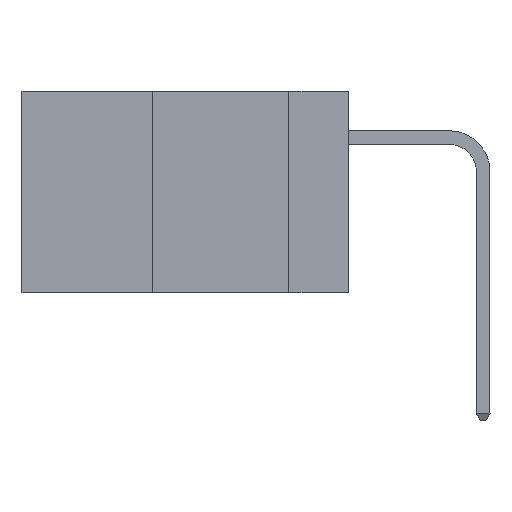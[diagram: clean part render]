
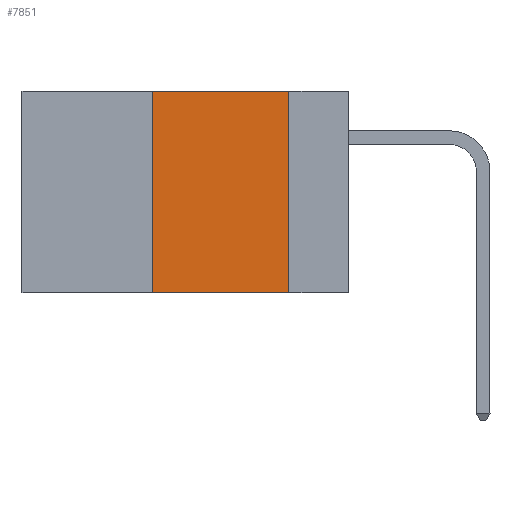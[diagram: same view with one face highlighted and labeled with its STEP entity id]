
A CAD part, left-side view. The second image highlights one B-rep face of the part: STEP entity #7851.
In plain terms, the highlighted planar face has unit normal (-1, 0, 0).
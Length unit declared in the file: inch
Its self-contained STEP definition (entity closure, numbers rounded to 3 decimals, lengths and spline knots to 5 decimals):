
#49 = CARTESIAN_POINT ( 'NONE',  ( 0., 0.36, 0. ) ) ;
#165 = DIRECTION ( 'NONE',  ( 0., 0., -1. ) ) ;
#714 = VERTEX_POINT ( 'NONE', #6493 ) ;
#869 = EDGE_CURVE ( 'NONE', #5033, #11792, #12158, .T. ) ;
#1617 = VECTOR ( 'NONE', #4748, 39.37008 ) ;
#1716 = ORIENTED_EDGE ( 'NONE', *, *, #869, .F. ) ;
#2442 = VECTOR ( 'NONE', #165, 39.37008 ) ;
#2627 = CARTESIAN_POINT ( 'NONE',  ( 0., 0.6, 0. ) ) ;
#3353 = FACE_OUTER_BOUND ( 'NONE', #8338, .T. ) ;
#3360 = EDGE_CURVE ( 'NONE', #11792, #714, #8730, .T. ) ;
#3423 = DIRECTION ( 'NONE',  ( 0., 0., -1. ) ) ;
#3955 = ORIENTED_EDGE ( 'NONE', *, *, #3360, .F. ) ;
#4748 = DIRECTION ( 'NONE',  ( 0., 0., 1. ) ) ;
#4960 = ORIENTED_EDGE ( 'NONE', *, *, #11251, .T. ) ;
#5033 = VERTEX_POINT ( 'NONE', #8714 ) ;
#5670 = CARTESIAN_POINT ( 'NONE',  ( 0., 0.11, -0.37 ) ) ;
#6016 = AXIS2_PLACEMENT_3D ( 'NONE', #8682, #12913, #3423 ) ;
#6493 = CARTESIAN_POINT ( 'NONE',  ( 0., 0.11, 0. ) ) ;
#6862 = VERTEX_POINT ( 'NONE', #5670 ) ;
#6981 = CARTESIAN_POINT ( 'NONE',  ( 0., 0.36, 0. ) ) ;
#7060 = ORIENTED_EDGE ( 'NONE', *, *, #13546, .F. ) ;
#7851 = ADVANCED_FACE ( 'NONE', ( #3353 ), #9721, .F. ) ;
#8328 = CARTESIAN_POINT ( 'NONE',  ( 0., 0.6, -0.37 ) ) ;
#8338 = EDGE_LOOP ( 'NONE', ( #7060, #3955, #1716, #4960 ) ) ;
#8682 = CARTESIAN_POINT ( 'NONE',  ( 0., 0.6, 0. ) ) ;
#8714 = CARTESIAN_POINT ( 'NONE',  ( 0., 0.36, -0.37 ) ) ;
#8730 = LINE ( 'NONE', #2627, #9589 ) ;
#9151 = LINE ( 'NONE', #8328, #11367 ) ;
#9589 = VECTOR ( 'NONE', #12961, 39.37008 ) ;
#9592 = CARTESIAN_POINT ( 'NONE',  ( 0., 0.11, 0. ) ) ;
#9721 = PLANE ( 'NONE',  #6016 ) ;
#11251 = EDGE_CURVE ( 'NONE', #5033, #6862, #9151, .T. ) ;
#11367 = VECTOR ( 'NONE', #12346, 39.37008 ) ;
#11679 = LINE ( 'NONE', #9592, #2442 ) ;
#11792 = VERTEX_POINT ( 'NONE', #49 ) ;
#12158 = LINE ( 'NONE', #6981, #1617 ) ;
#12346 = DIRECTION ( 'NONE',  ( 0., -1., 0. ) ) ;
#12913 = DIRECTION ( 'NONE',  ( 1., 0., 0. ) ) ;
#12961 = DIRECTION ( 'NONE',  ( 0., -1., 0. ) ) ;
#13546 = EDGE_CURVE ( 'NONE', #714, #6862, #11679, .T. ) ;
